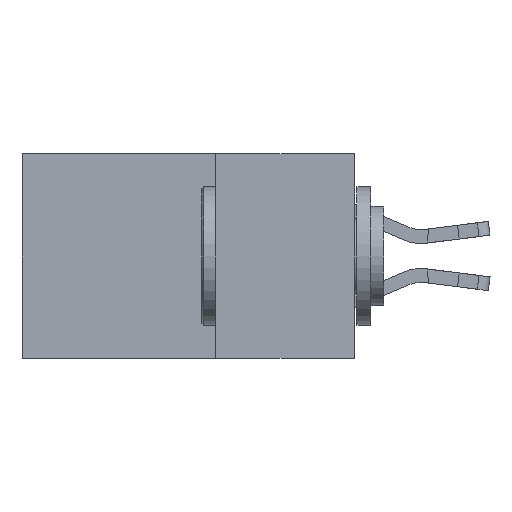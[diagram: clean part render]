
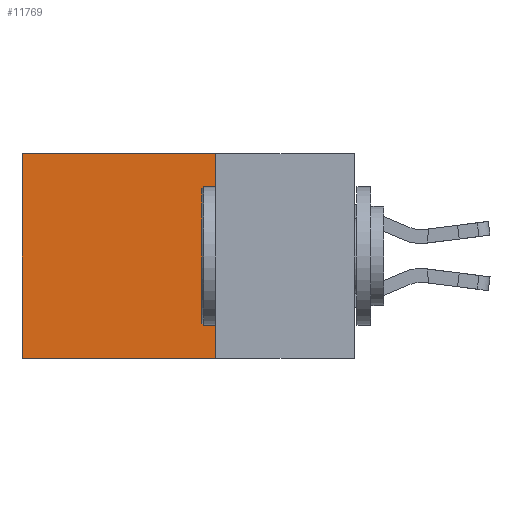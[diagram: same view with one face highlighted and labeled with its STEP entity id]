
A CAD part, left-side view. The second image highlights one B-rep face of the part: STEP entity #11769.
In plain terms, the highlighted planar face has unit normal (-1, 0, 0).
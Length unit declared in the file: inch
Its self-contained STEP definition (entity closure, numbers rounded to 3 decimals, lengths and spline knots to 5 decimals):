
#71 = DIRECTION ( 'NONE',  ( 0., 1., 0. ) ) ;
#480 = CARTESIAN_POINT ( 'NONE',  ( 0.2615, 0.25, -0.37 ) ) ;
#726 = LINE ( 'NONE', #7269, #18446 ) ;
#1655 = FACE_OUTER_BOUND ( 'NONE', #9695, .T. ) ;
#3048 = CARTESIAN_POINT ( 'NONE',  ( 0.2615, 0.25, -0.37 ) ) ;
#3094 = VECTOR ( 'NONE', #17258, 39.37008 ) ;
#5906 = CARTESIAN_POINT ( 'NONE',  ( 0.2615, 0.6, -0.37 ) ) ;
#5952 = ORIENTED_EDGE ( 'NONE', *, *, #10023, .T. ) ;
#5966 = DIRECTION ( 'NONE',  ( 0., 0., -1. ) ) ;
#6638 = VERTEX_POINT ( 'NONE', #18755 ) ;
#6722 = EDGE_CURVE ( 'NONE', #20782, #19779, #17140, .T. ) ;
#7269 = CARTESIAN_POINT ( 'NONE',  ( 0.2615, 0.6, -0.37 ) ) ;
#7822 = VECTOR ( 'NONE', #71, 39.37008 ) ;
#8077 = EDGE_CURVE ( 'NONE', #6638, #19779, #726, .T. ) ;
#9695 = EDGE_LOOP ( 'NONE', ( #13848, #14866, #12735, #5952 ) ) ;
#9750 = VECTOR ( 'NONE', #19987, 39.37008 ) ;
#10023 = EDGE_CURVE ( 'NONE', #12144, #6638, #12001, .T. ) ;
#10699 = CARTESIAN_POINT ( 'NONE',  ( 0.2615, 0.25, 0. ) ) ;
#11180 = CARTESIAN_POINT ( 'NONE',  ( 0.2615, 0.25, -0.37 ) ) ;
#11769 = ADVANCED_FACE ( 'NONE', ( #1655 ), #19995, .F. ) ;
#12001 = LINE ( 'NONE', #10699, #7822 ) ;
#12144 = VERTEX_POINT ( 'NONE', #21096 ) ;
#12735 = ORIENTED_EDGE ( 'NONE', *, *, #22588, .F. ) ;
#13733 = CARTESIAN_POINT ( 'NONE',  ( 0.2615, 0.25, -0.37 ) ) ;
#13848 = ORIENTED_EDGE ( 'NONE', *, *, #8077, .T. ) ;
#14014 = AXIS2_PLACEMENT_3D ( 'NONE', #11180, #16511, #5966 ) ;
#14866 = ORIENTED_EDGE ( 'NONE', *, *, #6722, .F. ) ;
#15014 = LINE ( 'NONE', #480, #9750 ) ;
#16511 = DIRECTION ( 'NONE',  ( 1., 0., 0. ) ) ;
#17140 = LINE ( 'NONE', #13733, #3094 ) ;
#17258 = DIRECTION ( 'NONE',  ( 0., 1., 0. ) ) ;
#18446 = VECTOR ( 'NONE', #21420, 39.37008 ) ;
#18755 = CARTESIAN_POINT ( 'NONE',  ( 0.2615, 0.6, 0. ) ) ;
#19779 = VERTEX_POINT ( 'NONE', #5906 ) ;
#19987 = DIRECTION ( 'NONE',  ( 0., 0., -1. ) ) ;
#19995 = PLANE ( 'NONE',  #14014 ) ;
#20782 = VERTEX_POINT ( 'NONE', #3048 ) ;
#21096 = CARTESIAN_POINT ( 'NONE',  ( 0.2615, 0.25, 0. ) ) ;
#21420 = DIRECTION ( 'NONE',  ( 0., 0., -1. ) ) ;
#22588 = EDGE_CURVE ( 'NONE', #12144, #20782, #15014, .T. ) ;
